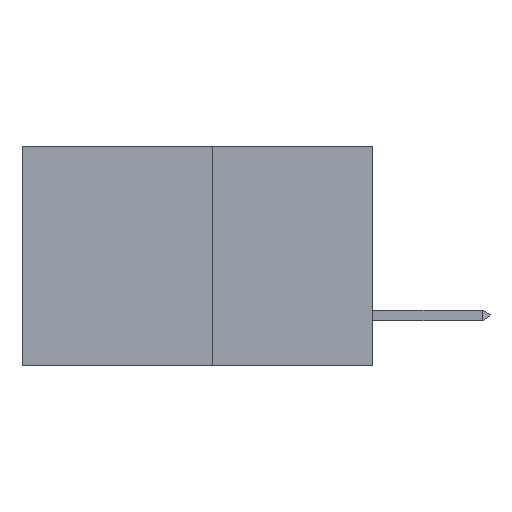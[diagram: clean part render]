
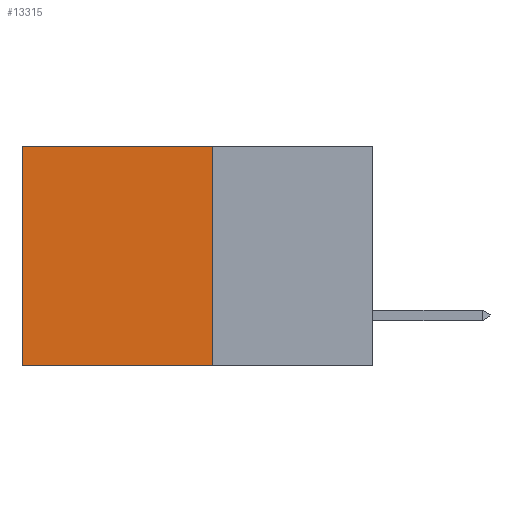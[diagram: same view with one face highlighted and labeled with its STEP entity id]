
A CAD part, left-side view. The second image highlights one B-rep face of the part: STEP entity #13315.
In plain terms, the highlighted planar face has unit normal (-1, 0, 0).
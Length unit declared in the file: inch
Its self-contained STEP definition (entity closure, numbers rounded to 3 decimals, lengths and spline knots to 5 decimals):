
#188 = EDGE_LOOP ( 'NONE', ( #15542, #4408, #5332, #13112 ) ) ;
#368 = VERTEX_POINT ( 'NONE', #7349 ) ;
#898 = DIRECTION ( 'NONE',  ( 0., 0., -1. ) ) ;
#910 = DIRECTION ( 'NONE',  ( 0., 1., 0. ) ) ;
#954 = CARTESIAN_POINT ( 'NONE',  ( 0.277, 0.27, 0. ) ) ;
#2562 = VERTEX_POINT ( 'NONE', #3659 ) ;
#3399 = FACE_OUTER_BOUND ( 'NONE', #188, .T. ) ;
#3659 = CARTESIAN_POINT ( 'NONE',  ( 0.277, 0.27, -0.37 ) ) ;
#4098 = VERTEX_POINT ( 'NONE', #13581 ) ;
#4342 = LINE ( 'NONE', #12649, #7324 ) ;
#4408 = ORIENTED_EDGE ( 'NONE', *, *, #16147, .F. ) ;
#4629 = LINE ( 'NONE', #8726, #11097 ) ;
#5177 = VECTOR ( 'NONE', #8595, 39.37008 ) ;
#5332 = ORIENTED_EDGE ( 'NONE', *, *, #16220, .F. ) ;
#5590 = EDGE_CURVE ( 'NONE', #14504, #368, #4629, .T. ) ;
#7324 = VECTOR ( 'NONE', #898, 39.37008 ) ;
#7349 = CARTESIAN_POINT ( 'NONE',  ( 0.277, 0.59, 0. ) ) ;
#7612 = DIRECTION ( 'NONE',  ( 0., 0., -1. ) ) ;
#7680 = CARTESIAN_POINT ( 'NONE',  ( 0.277, 0.27, -0.37 ) ) ;
#8595 = DIRECTION ( 'NONE',  ( 0., 1., 0. ) ) ;
#8726 = CARTESIAN_POINT ( 'NONE',  ( 0.277, 0.27, 0. ) ) ;
#8978 = DIRECTION ( 'NONE',  ( 0., 0., -1. ) ) ;
#11097 = VECTOR ( 'NONE', #910, 39.37008 ) ;
#12427 = VECTOR ( 'NONE', #7612, 39.37008 ) ;
#12649 = CARTESIAN_POINT ( 'NONE',  ( 0.277, 0.27, -0.37 ) ) ;
#12810 = LINE ( 'NONE', #14030, #12427 ) ;
#13112 = ORIENTED_EDGE ( 'NONE', *, *, #5590, .T. ) ;
#13315 = ADVANCED_FACE ( 'NONE', ( #3399 ), #15358, .F. ) ;
#13581 = CARTESIAN_POINT ( 'NONE',  ( 0.277, 0.59, -0.37 ) ) ;
#13752 = CARTESIAN_POINT ( 'NONE',  ( 0.277, 0.27, -0.37 ) ) ;
#14030 = CARTESIAN_POINT ( 'NONE',  ( 0.277, 0.59, -0.37 ) ) ;
#14504 = VERTEX_POINT ( 'NONE', #954 ) ;
#15358 = PLANE ( 'NONE',  #15559 ) ;
#15542 = ORIENTED_EDGE ( 'NONE', *, *, #15707, .T. ) ;
#15559 = AXIS2_PLACEMENT_3D ( 'NONE', #7680, #16566, #8978 ) ;
#15707 = EDGE_CURVE ( 'NONE', #368, #4098, #12810, .T. ) ;
#15721 = LINE ( 'NONE', #13752, #5177 ) ;
#16147 = EDGE_CURVE ( 'NONE', #2562, #4098, #15721, .T. ) ;
#16220 = EDGE_CURVE ( 'NONE', #14504, #2562, #4342, .T. ) ;
#16566 = DIRECTION ( 'NONE',  ( 1., 0., 0. ) ) ;
